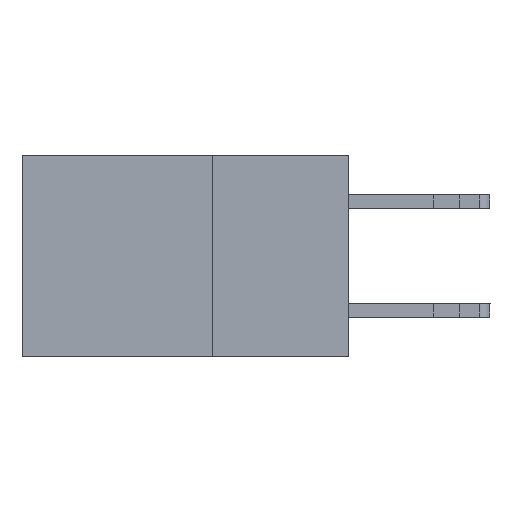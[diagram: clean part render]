
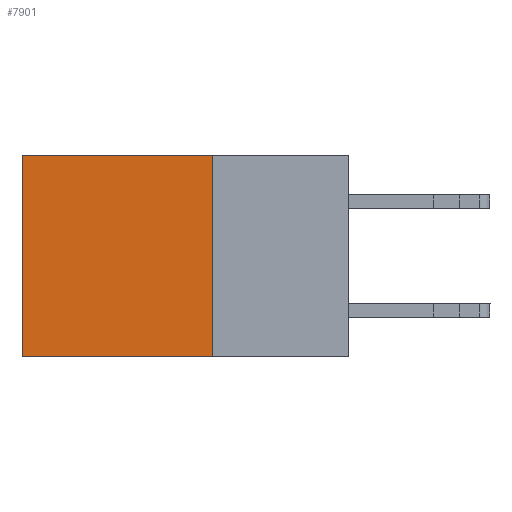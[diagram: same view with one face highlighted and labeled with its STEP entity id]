
A CAD part, left-side view. The second image highlights one B-rep face of the part: STEP entity #7901.
In plain terms, the highlighted planar face has unit normal (-1, 0, 0).
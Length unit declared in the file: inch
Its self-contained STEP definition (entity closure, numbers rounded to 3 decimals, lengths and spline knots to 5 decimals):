
#809 = VERTEX_POINT ( 'NONE', #3621 ) ;
#1122 = DIRECTION ( 'NONE',  ( 1., 0., 0. ) ) ;
#1881 = VECTOR ( 'NONE', #8812, 39.37008 ) ;
#2409 = EDGE_LOOP ( 'NONE', ( #25427, #7411, #12845, #3696 ) ) ;
#2473 = CARTESIAN_POINT ( 'NONE',  ( 0.298, 0.25, -0.37 ) ) ;
#3621 = CARTESIAN_POINT ( 'NONE',  ( 0.298, 0.6, -0.37 ) ) ;
#3696 = ORIENTED_EDGE ( 'NONE', *, *, #24879, .T. ) ;
#3777 = DIRECTION ( 'NONE',  ( 0., 0., -1. ) ) ;
#4294 = EDGE_CURVE ( 'NONE', #11721, #809, #23936, .T. ) ;
#4839 = EDGE_CURVE ( 'NONE', #20111, #809, #8791, .T. ) ;
#7411 = ORIENTED_EDGE ( 'NONE', *, *, #4294, .F. ) ;
#7529 = CARTESIAN_POINT ( 'NONE',  ( 0.298, 0.25, -0.37 ) ) ;
#7901 = ADVANCED_FACE ( 'NONE', ( #23654 ), #17654, .F. ) ;
#8649 = DIRECTION ( 'NONE',  ( 0., 1., 0. ) ) ;
#8791 = LINE ( 'NONE', #12764, #1881 ) ;
#8812 = DIRECTION ( 'NONE',  ( 0., 0., -1. ) ) ;
#10584 = CARTESIAN_POINT ( 'NONE',  ( 0.298, 0.25, 0. ) ) ;
#11358 = CARTESIAN_POINT ( 'NONE',  ( 0.298, 0.25, 0. ) ) ;
#11721 = VERTEX_POINT ( 'NONE', #2473 ) ;
#12627 = LINE ( 'NONE', #13810, #17523 ) ;
#12764 = CARTESIAN_POINT ( 'NONE',  ( 0.298, 0.6, 0. ) ) ;
#12845 = ORIENTED_EDGE ( 'NONE', *, *, #18327, .F. ) ;
#13761 = DIRECTION ( 'NONE',  ( 0., 1., 0. ) ) ;
#13810 = CARTESIAN_POINT ( 'NONE',  ( 0.298, 0.25, 0. ) ) ;
#17523 = VECTOR ( 'NONE', #24359, 39.37008 ) ;
#17654 = PLANE ( 'NONE',  #27074 ) ;
#18327 = EDGE_CURVE ( 'NONE', #18552, #11721, #12627, .T. ) ;
#18552 = VERTEX_POINT ( 'NONE', #22902 ) ;
#19201 = CARTESIAN_POINT ( 'NONE',  ( 0.298, 0.6, 0. ) ) ;
#20111 = VERTEX_POINT ( 'NONE', #19201 ) ;
#22902 = CARTESIAN_POINT ( 'NONE',  ( 0.298, 0.25, 0. ) ) ;
#23154 = LINE ( 'NONE', #10584, #23805 ) ;
#23654 = FACE_OUTER_BOUND ( 'NONE', #2409, .T. ) ;
#23805 = VECTOR ( 'NONE', #8649, 39.37008 ) ;
#23936 = LINE ( 'NONE', #7529, #26905 ) ;
#24359 = DIRECTION ( 'NONE',  ( 0., 0., -1. ) ) ;
#24879 = EDGE_CURVE ( 'NONE', #18552, #20111, #23154, .T. ) ;
#25427 = ORIENTED_EDGE ( 'NONE', *, *, #4839, .T. ) ;
#26905 = VECTOR ( 'NONE', #13761, 39.37008 ) ;
#27074 = AXIS2_PLACEMENT_3D ( 'NONE', #11358, #1122, #3777 ) ;
